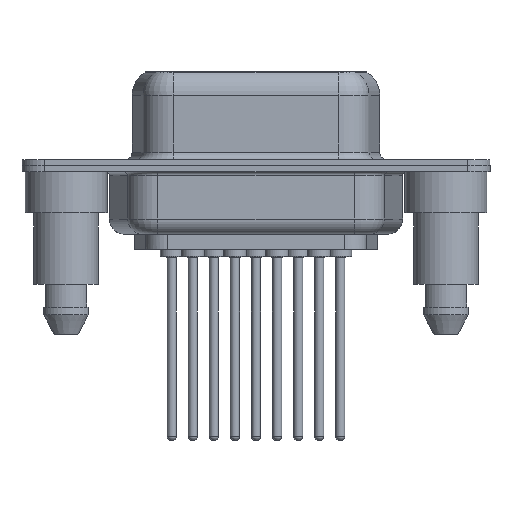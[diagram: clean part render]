
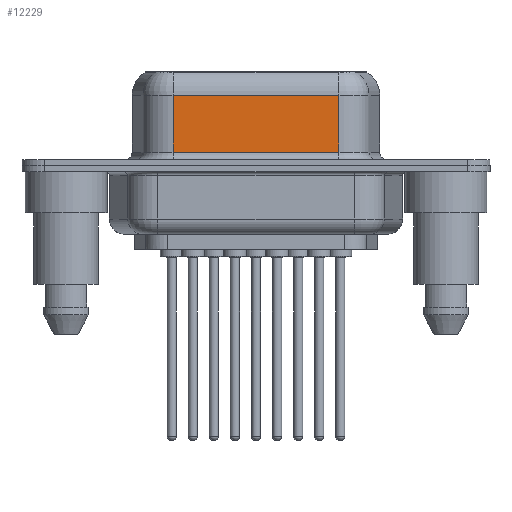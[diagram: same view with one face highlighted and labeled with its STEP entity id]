
A CAD part, front view. The second image highlights one B-rep face of the part: STEP entity #12229.
In plain terms, the highlighted planar face has unit normal (0, -1, 0).
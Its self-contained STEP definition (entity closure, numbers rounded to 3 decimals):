
#877 = DIRECTION ( 'NONE',  ( 0., 1., 0. ) ) ;
#957 = DIRECTION ( 'NONE',  ( 0., 0., 1. ) ) ;
#1037 = CARTESIAN_POINT ( 'NONE',  ( 7.038, -3.95, 4.65 ) ) ;
#1166 = VERTEX_POINT ( 'NONE', #9356 ) ;
#1562 = LINE ( 'NONE', #15418, #8435 ) ;
#2133 = PLANE ( 'NONE',  #12181 ) ;
#2589 = EDGE_LOOP ( 'NONE', ( #3212, #7791, #12114, #9276 ) ) ;
#2664 = VECTOR ( 'NONE', #6702, 1000. ) ;
#2715 = DIRECTION ( 'NONE',  ( 0., 0., -1. ) ) ;
#3212 = ORIENTED_EDGE ( 'NONE', *, *, #7224, .F. ) ;
#5258 = EDGE_CURVE ( 'NONE', #1166, #14523, #1562, .T. ) ;
#6193 = VERTEX_POINT ( 'NONE', #12304 ) ;
#6702 = DIRECTION ( 'NONE',  ( 1., 0., 0. ) ) ;
#7224 = EDGE_CURVE ( 'NONE', #1166, #15164, #12717, .T. ) ;
#7742 = DIRECTION ( 'NONE',  ( -1., 0., 0. ) ) ;
#7791 = ORIENTED_EDGE ( 'NONE', *, *, #5258, .T. ) ;
#8435 = VECTOR ( 'NONE', #7742, 1000. ) ;
#9271 = VECTOR ( 'NONE', #2715, 1000. ) ;
#9276 = ORIENTED_EDGE ( 'NONE', *, *, #14558, .T. ) ;
#9356 = CARTESIAN_POINT ( 'NONE',  ( 17.962, -3.95, 4.65 ) ) ;
#11488 = CARTESIAN_POINT ( 'NONE',  ( 17.962, -3.95, 6.4 ) ) ;
#11593 = LINE ( 'NONE', #15715, #2664 ) ;
#11924 = CARTESIAN_POINT ( 'NONE',  ( 7.038, -3.95, 6.4 ) ) ;
#12114 = ORIENTED_EDGE ( 'NONE', *, *, #14642, .T. ) ;
#12181 = AXIS2_PLACEMENT_3D ( 'NONE', #12349, #877, #957 ) ;
#12229 = ADVANCED_FACE ( 'NONE', ( #14652 ), #2133, .F. ) ;
#12304 = CARTESIAN_POINT ( 'NONE',  ( 7.038, -3.95, 0.9 ) ) ;
#12319 = CARTESIAN_POINT ( 'NONE',  ( 17.962, -3.95, 0.9 ) ) ;
#12349 = CARTESIAN_POINT ( 'NONE',  ( 17.962, -3.95, 6.4 ) ) ;
#12520 = VECTOR ( 'NONE', #15269, 1000. ) ;
#12717 = LINE ( 'NONE', #11488, #12520 ) ;
#14218 = LINE ( 'NONE', #11924, #9271 ) ;
#14523 = VERTEX_POINT ( 'NONE', #1037 ) ;
#14558 = EDGE_CURVE ( 'NONE', #6193, #15164, #11593, .T. ) ;
#14642 = EDGE_CURVE ( 'NONE', #14523, #6193, #14218, .T. ) ;
#14652 = FACE_OUTER_BOUND ( 'NONE', #2589, .T. ) ;
#15164 = VERTEX_POINT ( 'NONE', #12319 ) ;
#15269 = DIRECTION ( 'NONE',  ( 0., 0., -1. ) ) ;
#15418 = CARTESIAN_POINT ( 'NONE',  ( 17.962, -3.95, 4.65 ) ) ;
#15715 = CARTESIAN_POINT ( 'NONE',  ( 17.962, -3.95, 0.9 ) ) ;
